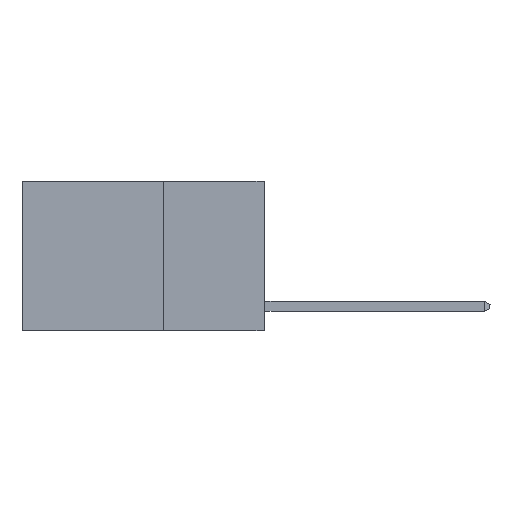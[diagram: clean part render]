
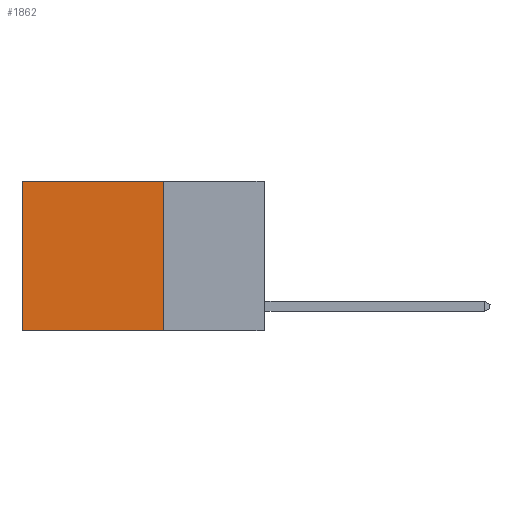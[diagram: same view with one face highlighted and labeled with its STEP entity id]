
A CAD part, left-side view. The second image highlights one B-rep face of the part: STEP entity #1862.
In plain terms, the highlighted planar face has unit normal (-1, 0, 0).
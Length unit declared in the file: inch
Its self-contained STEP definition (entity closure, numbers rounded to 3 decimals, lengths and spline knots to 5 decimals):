
#880 = DIRECTION ( 'NONE',  ( 0., 0., -1. ) ) ;
#1433 = VERTEX_POINT ( 'NONE', #15774 ) ;
#1539 = LINE ( 'NONE', #16586, #15579 ) ;
#1862 = ADVANCED_FACE ( 'NONE', ( #6540 ), #15876, .F. ) ;
#2021 = VERTEX_POINT ( 'NONE', #3095 ) ;
#2094 = ORIENTED_EDGE ( 'NONE', *, *, #8276, .F. ) ;
#2586 = VERTEX_POINT ( 'NONE', #15973 ) ;
#2837 = CARTESIAN_POINT ( 'NONE',  ( 0.2625, 0.6, 0. ) ) ;
#3095 = CARTESIAN_POINT ( 'NONE',  ( 0.2625, 0.25, -0.37 ) ) ;
#3307 = LINE ( 'NONE', #6317, #10283 ) ;
#3952 = CARTESIAN_POINT ( 'NONE',  ( 0.2625, 0.25, 0. ) ) ;
#4108 = DIRECTION ( 'NONE',  ( 0., 1., 0. ) ) ;
#4916 = DIRECTION ( 'NONE',  ( 0., 1., 0. ) ) ;
#5710 = EDGE_CURVE ( 'NONE', #1433, #14457, #12437, .T. ) ;
#6317 = CARTESIAN_POINT ( 'NONE',  ( 0.2625, 0.25, -0.37 ) ) ;
#6405 = ORIENTED_EDGE ( 'NONE', *, *, #12637, .T. ) ;
#6540 = FACE_OUTER_BOUND ( 'NONE', #10989, .T. ) ;
#8071 = VECTOR ( 'NONE', #10449, 39.37008 ) ;
#8184 = DIRECTION ( 'NONE',  ( 0., 0., -1. ) ) ;
#8276 = EDGE_CURVE ( 'NONE', #1433, #2021, #1539, .T. ) ;
#10283 = VECTOR ( 'NONE', #4916, 39.37008 ) ;
#10449 = DIRECTION ( 'NONE',  ( 0., 0., -1. ) ) ;
#10524 = AXIS2_PLACEMENT_3D ( 'NONE', #15997, #11951, #8184 ) ;
#10579 = EDGE_CURVE ( 'NONE', #2021, #2586, #3307, .T. ) ;
#10989 = EDGE_LOOP ( 'NONE', ( #6405, #12285, #2094, #15491 ) ) ;
#11358 = LINE ( 'NONE', #16842, #8071 ) ;
#11951 = DIRECTION ( 'NONE',  ( 1., 0., 0. ) ) ;
#12285 = ORIENTED_EDGE ( 'NONE', *, *, #10579, .F. ) ;
#12437 = LINE ( 'NONE', #3952, #13413 ) ;
#12637 = EDGE_CURVE ( 'NONE', #14457, #2586, #11358, .T. ) ;
#13413 = VECTOR ( 'NONE', #4108, 39.37008 ) ;
#14457 = VERTEX_POINT ( 'NONE', #2837 ) ;
#15491 = ORIENTED_EDGE ( 'NONE', *, *, #5710, .T. ) ;
#15579 = VECTOR ( 'NONE', #880, 39.37008 ) ;
#15774 = CARTESIAN_POINT ( 'NONE',  ( 0.2625, 0.25, 0. ) ) ;
#15876 = PLANE ( 'NONE',  #10524 ) ;
#15973 = CARTESIAN_POINT ( 'NONE',  ( 0.2625, 0.6, -0.37 ) ) ;
#15997 = CARTESIAN_POINT ( 'NONE',  ( 0.2625, 0.25, 0. ) ) ;
#16586 = CARTESIAN_POINT ( 'NONE',  ( 0.2625, 0.25, 0. ) ) ;
#16842 = CARTESIAN_POINT ( 'NONE',  ( 0.2625, 0.6, 0. ) ) ;
